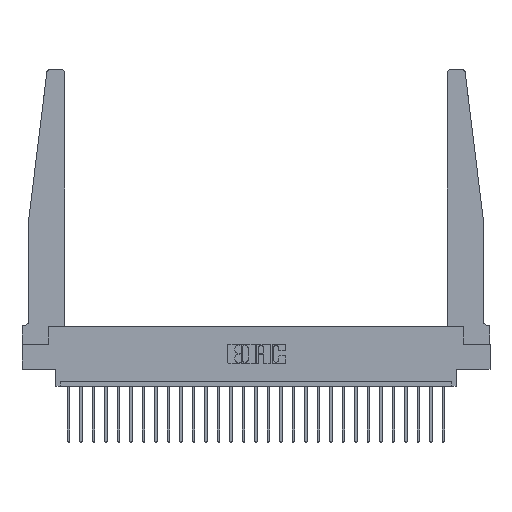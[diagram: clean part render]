
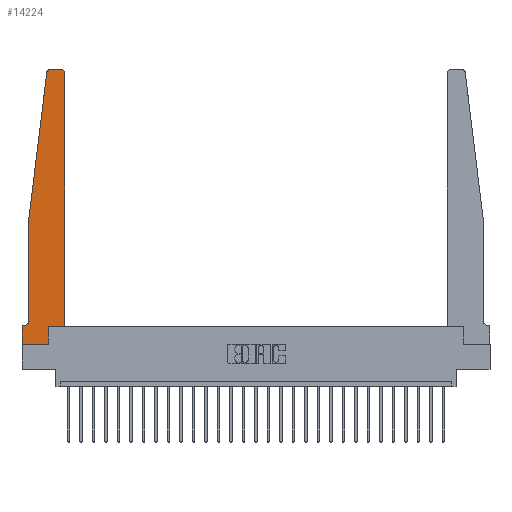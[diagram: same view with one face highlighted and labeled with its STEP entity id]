
A CAD part, top view. The second image highlights one B-rep face of the part: STEP entity #14224.
In plain terms, the highlighted planar face has unit normal (0, 0, 1).
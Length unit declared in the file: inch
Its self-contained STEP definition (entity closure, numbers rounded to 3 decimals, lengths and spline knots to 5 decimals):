
#5 = CARTESIAN_POINT ( 'NONE',  ( 0.395, 2.72, 0.37 ) ) ;
#129 = DIRECTION ( 'NONE',  ( -0.122, -0.992, 0. ) ) ;
#539 = VERTEX_POINT ( 'NONE', #8942 ) ;
#871 = EDGE_CURVE ( 'NONE', #13604, #10709, #5983, .T. ) ;
#1664 = FACE_OUTER_BOUND ( 'NONE', #11099, .T. ) ;
#1666 = CARTESIAN_POINT ( 'NONE',  ( 0., 0., 0.37 ) ) ;
#1842 = CARTESIAN_POINT ( 'NONE',  ( 0., 0., 0.37 ) ) ;
#1907 = ORIENTED_EDGE ( 'NONE', *, *, #3818, .T. ) ;
#2166 = CARTESIAN_POINT ( 'NONE',  ( 0.425, 2.72, 0.37 ) ) ;
#2710 = VECTOR ( 'NONE', #14028, 39.37008 ) ;
#2927 = ORIENTED_EDGE ( 'NONE', *, *, #4458, .T. ) ;
#2948 = DIRECTION ( 'NONE',  ( -1., 0., 0. ) ) ;
#3054 = CARTESIAN_POINT ( 'NONE',  ( 0.065, 1.25, 0.37 ) ) ;
#3175 = VECTOR ( 'NONE', #129, 39.37008 ) ;
#3371 = DIRECTION ( 'NONE',  ( 1., 0., 0. ) ) ;
#3482 = DIRECTION ( 'NONE',  ( 0., 1., 0. ) ) ;
#3561 = CARTESIAN_POINT ( 'NONE',  ( 0.065, 1.25, 0.37 ) ) ;
#3794 = DIRECTION ( 'NONE',  ( 0., -1., 0. ) ) ;
#3818 = EDGE_CURVE ( 'NONE', #13889, #539, #25858, .T. ) ;
#4061 = PLANE ( 'NONE',  #17504 ) ;
#4309 = VECTOR ( 'NONE', #3482, 39.37008 ) ;
#4458 = EDGE_CURVE ( 'NONE', #16571, #13604, #21124, .T. ) ;
#4682 = DIRECTION ( 'NONE',  ( 0., 0., -1. ) ) ;
#5212 = LINE ( 'NONE', #21167, #21711 ) ;
#5314 = VERTEX_POINT ( 'NONE', #8456 ) ;
#5820 = EDGE_CURVE ( 'NONE', #7093, #23375, #6194, .T. ) ;
#5832 = DIRECTION ( 'NONE',  ( -1., 0., 0. ) ) ;
#5876 = ORIENTED_EDGE ( 'NONE', *, *, #13218, .T. ) ;
#5983 = CIRCLE ( 'NONE', #25755, 0.05 ) ;
#6170 = AXIS2_PLACEMENT_3D ( 'NONE', #5, #6463, #16610 ) ;
#6194 = CIRCLE ( 'NONE', #8305, 0.03 ) ;
#6432 = DIRECTION ( 'NONE',  ( 0., 0., 1. ) ) ;
#6463 = DIRECTION ( 'NONE',  ( 0., 0., 1. ) ) ;
#6483 = CARTESIAN_POINT ( 'NONE',  ( 0.065, 0.1875, 0.37 ) ) ;
#6994 = CIRCLE ( 'NONE', #6170, 0.03 ) ;
#7093 = VERTEX_POINT ( 'NONE', #20935 ) ;
#7565 = CARTESIAN_POINT ( 'NONE',  ( 0.2605, 0.18, 0.37 ) ) ;
#8305 = AXIS2_PLACEMENT_3D ( 'NONE', #14492, #6432, #10369 ) ;
#8456 = CARTESIAN_POINT ( 'NONE',  ( 0.425, 0.18, 0.37 ) ) ;
#8539 = CARTESIAN_POINT ( 'NONE',  ( 0.395, 2.75, 0.37 ) ) ;
#8942 = CARTESIAN_POINT ( 'NONE',  ( 0.2605, 0., 0.37 ) ) ;
#9179 = CARTESIAN_POINT ( 'NONE',  ( 0.24675, 2.72367, 0.37 ) ) ;
#9293 = ORIENTED_EDGE ( 'NONE', *, *, #17214, .T. ) ;
#9381 = LINE ( 'NONE', #17438, #11608 ) ;
#9855 = ORIENTED_EDGE ( 'NONE', *, *, #25903, .T. ) ;
#10171 = EDGE_CURVE ( 'NONE', #22450, #13889, #17657, .T. ) ;
#10369 = DIRECTION ( 'NONE',  ( 1., 0., 0. ) ) ;
#10709 = VERTEX_POINT ( 'NONE', #13918 ) ;
#10710 = CARTESIAN_POINT ( 'NONE',  ( 0.015, 0.2375, 0.37 ) ) ;
#10748 = CARTESIAN_POINT ( 'NONE',  ( 0.065, 1.25, 0.37 ) ) ;
#11099 = EDGE_LOOP ( 'NONE', ( #5876, #18106, #9855, #2927, #18055, #20648, #20513, #1907, #12695, #13807, #11918, #9293 ) ) ;
#11608 = VECTOR ( 'NONE', #5832, 39.37008 ) ;
#11660 = VERTEX_POINT ( 'NONE', #8539 ) ;
#11918 = ORIENTED_EDGE ( 'NONE', *, *, #15277, .T. ) ;
#12243 = EDGE_CURVE ( 'NONE', #539, #16389, #21552, .T. ) ;
#12695 = ORIENTED_EDGE ( 'NONE', *, *, #12243, .T. ) ;
#13218 = EDGE_CURVE ( 'NONE', #11660, #7093, #9381, .T. ) ;
#13604 = VERTEX_POINT ( 'NONE', #25700 ) ;
#13807 = ORIENTED_EDGE ( 'NONE', *, *, #24940, .T. ) ;
#13889 = VERTEX_POINT ( 'NONE', #15018 ) ;
#13918 = CARTESIAN_POINT ( 'NONE',  ( 0.015, 0.1875, 0.37 ) ) ;
#13949 = DIRECTION ( 'NONE',  ( 1., 0., 0. ) ) ;
#14028 = DIRECTION ( 'NONE',  ( -1., 0., 0. ) ) ;
#14224 = ADVANCED_FACE ( 'NONE', ( #1664 ), #4061, .T. ) ;
#14492 = CARTESIAN_POINT ( 'NONE',  ( 0.27653, 2.72, 0.37 ) ) ;
#14670 = CARTESIAN_POINT ( 'NONE',  ( 0., 0.1875, 0.37 ) ) ;
#15018 = CARTESIAN_POINT ( 'NONE',  ( 0., 0., 0.37 ) ) ;
#15277 = EDGE_CURVE ( 'NONE', #5314, #25097, #23832, .T. ) ;
#15926 = DIRECTION ( 'NONE',  ( 0., 0., 1. ) ) ;
#16109 = VECTOR ( 'NONE', #3794, 39.37008 ) ;
#16327 = CARTESIAN_POINT ( 'NONE',  ( 0.2605, 0.18, 0.37 ) ) ;
#16389 = VERTEX_POINT ( 'NONE', #16327 ) ;
#16571 = VERTEX_POINT ( 'NONE', #10748 ) ;
#16610 = DIRECTION ( 'NONE',  ( 1., 0., 0. ) ) ;
#17029 = DIRECTION ( 'NONE',  ( 0., -1., 0. ) ) ;
#17214 = EDGE_CURVE ( 'NONE', #25097, #11660, #6994, .T. ) ;
#17438 = CARTESIAN_POINT ( 'NONE',  ( 0.25, 2.75, 0.37 ) ) ;
#17504 = AXIS2_PLACEMENT_3D ( 'NONE', #25938, #15926, #13949 ) ;
#17626 = VECTOR ( 'NONE', #21906, 39.37008 ) ;
#17657 = LINE ( 'NONE', #1666, #16109 ) ;
#18055 = ORIENTED_EDGE ( 'NONE', *, *, #871, .T. ) ;
#18106 = ORIENTED_EDGE ( 'NONE', *, *, #5820, .T. ) ;
#18402 = LINE ( 'NONE', #6483, #2710 ) ;
#20513 = ORIENTED_EDGE ( 'NONE', *, *, #10171, .T. ) ;
#20648 = ORIENTED_EDGE ( 'NONE', *, *, #22337, .T. ) ;
#20935 = CARTESIAN_POINT ( 'NONE',  ( 0.27653, 2.75, 0.37 ) ) ;
#21124 = LINE ( 'NONE', #3054, #25627 ) ;
#21167 = CARTESIAN_POINT ( 'NONE',  ( 0.425, 0.18, 0.37 ) ) ;
#21552 = LINE ( 'NONE', #7565, #4309 ) ;
#21711 = VECTOR ( 'NONE', #3371, 39.37008 ) ;
#21906 = DIRECTION ( 'NONE',  ( 1., 0., 0. ) ) ;
#22337 = EDGE_CURVE ( 'NONE', #10709, #22450, #18402, .T. ) ;
#22450 = VERTEX_POINT ( 'NONE', #14670 ) ;
#22579 = VECTOR ( 'NONE', #23966, 39.37008 ) ;
#23375 = VERTEX_POINT ( 'NONE', #9179 ) ;
#23832 = LINE ( 'NONE', #24361, #22579 ) ;
#23966 = DIRECTION ( 'NONE',  ( 0., 1., 0. ) ) ;
#24361 = CARTESIAN_POINT ( 'NONE',  ( 0.425, 0.18, 0.37 ) ) ;
#24940 = EDGE_CURVE ( 'NONE', #16389, #5314, #5212, .T. ) ;
#25097 = VERTEX_POINT ( 'NONE', #2166 ) ;
#25627 = VECTOR ( 'NONE', #17029, 39.37008 ) ;
#25700 = CARTESIAN_POINT ( 'NONE',  ( 0.065, 0.2375, 0.37 ) ) ;
#25755 = AXIS2_PLACEMENT_3D ( 'NONE', #10710, #4682, #2948 ) ;
#25838 = LINE ( 'NONE', #3561, #3175 ) ;
#25858 = LINE ( 'NONE', #1842, #17626 ) ;
#25903 = EDGE_CURVE ( 'NONE', #23375, #16571, #25838, .T. ) ;
#25938 = CARTESIAN_POINT ( 'NONE',  ( 0., 0.1875, 0.37 ) ) ;
